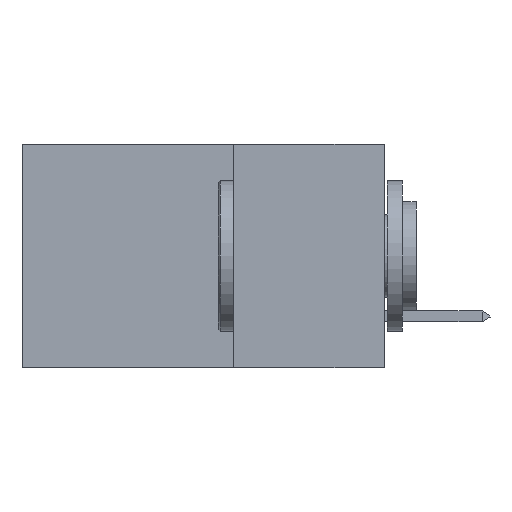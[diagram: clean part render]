
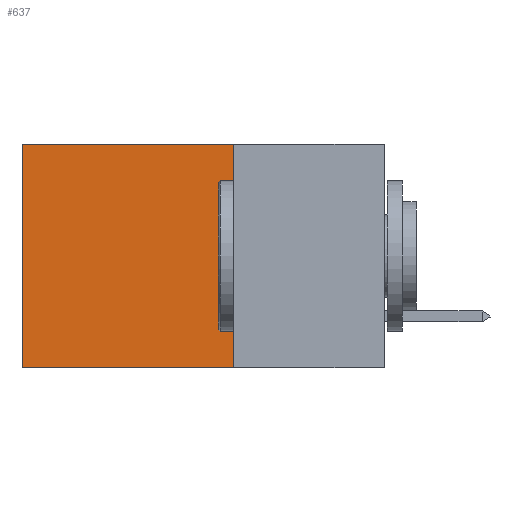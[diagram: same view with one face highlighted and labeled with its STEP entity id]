
A CAD part, left-side view. The second image highlights one B-rep face of the part: STEP entity #637.
In plain terms, the highlighted planar face has unit normal (-1, 0, 0).
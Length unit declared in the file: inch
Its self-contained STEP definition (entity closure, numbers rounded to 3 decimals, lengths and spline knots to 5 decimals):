
#33 = LINE ( 'NONE', #2863, #17476 ) ;
#424 = ORIENTED_EDGE ( 'NONE', *, *, #8582, .F. ) ;
#637 = ADVANCED_FACE ( 'NONE', ( #12572 ), #14891, .F. ) ;
#2863 = CARTESIAN_POINT ( 'NONE',  ( 0.2875, 0.6, 0. ) ) ;
#2972 = CARTESIAN_POINT ( 'NONE',  ( 0.2875, 0.6, -0.37 ) ) ;
#3028 = LINE ( 'NONE', #12488, #6290 ) ;
#3479 = AXIS2_PLACEMENT_3D ( 'NONE', #14957, #3932, #14755 ) ;
#3819 = LINE ( 'NONE', #12859, #20229 ) ;
#3932 = DIRECTION ( 'NONE',  ( 1., 0., 0. ) ) ;
#4379 = VERTEX_POINT ( 'NONE', #2972 ) ;
#5395 = EDGE_CURVE ( 'NONE', #18960, #12154, #6985, .T. ) ;
#6184 = ORIENTED_EDGE ( 'NONE', *, *, #12806, .F. ) ;
#6290 = VECTOR ( 'NONE', #19109, 39.37008 ) ;
#6967 = EDGE_LOOP ( 'NONE', ( #18208, #424, #6184, #9435 ) ) ;
#6985 = LINE ( 'NONE', #12907, #14901 ) ;
#8582 = EDGE_CURVE ( 'NONE', #17740, #4379, #3819, .T. ) ;
#9418 = CARTESIAN_POINT ( 'NONE',  ( 0.2875, 0.25, -0.37 ) ) ;
#9435 = ORIENTED_EDGE ( 'NONE', *, *, #5395, .T. ) ;
#9518 = DIRECTION ( 'NONE',  ( 0., 1., 0. ) ) ;
#11240 = CARTESIAN_POINT ( 'NONE',  ( 0.2875, 0.6, 0. ) ) ;
#12150 = DIRECTION ( 'NONE',  ( 0., 0., -1. ) ) ;
#12154 = VERTEX_POINT ( 'NONE', #11240 ) ;
#12488 = CARTESIAN_POINT ( 'NONE',  ( 0.2875, 0.25, 0. ) ) ;
#12572 = FACE_OUTER_BOUND ( 'NONE', #6967, .T. ) ;
#12806 = EDGE_CURVE ( 'NONE', #18960, #17740, #3028, .T. ) ;
#12859 = CARTESIAN_POINT ( 'NONE',  ( 0.2875, 0.25, -0.37 ) ) ;
#12907 = CARTESIAN_POINT ( 'NONE',  ( 0.2875, 0.25, 0. ) ) ;
#14368 = CARTESIAN_POINT ( 'NONE',  ( 0.2875, 0.25, 0. ) ) ;
#14755 = DIRECTION ( 'NONE',  ( 0., 0., -1. ) ) ;
#14829 = DIRECTION ( 'NONE',  ( 0., 1., 0. ) ) ;
#14891 = PLANE ( 'NONE',  #3479 ) ;
#14901 = VECTOR ( 'NONE', #14829, 39.37008 ) ;
#14957 = CARTESIAN_POINT ( 'NONE',  ( 0.2875, 0.25, 0. ) ) ;
#17476 = VECTOR ( 'NONE', #12150, 39.37008 ) ;
#17562 = EDGE_CURVE ( 'NONE', #12154, #4379, #33, .T. ) ;
#17740 = VERTEX_POINT ( 'NONE', #9418 ) ;
#18208 = ORIENTED_EDGE ( 'NONE', *, *, #17562, .T. ) ;
#18960 = VERTEX_POINT ( 'NONE', #14368 ) ;
#19109 = DIRECTION ( 'NONE',  ( 0., 0., -1. ) ) ;
#20229 = VECTOR ( 'NONE', #9518, 39.37008 ) ;
